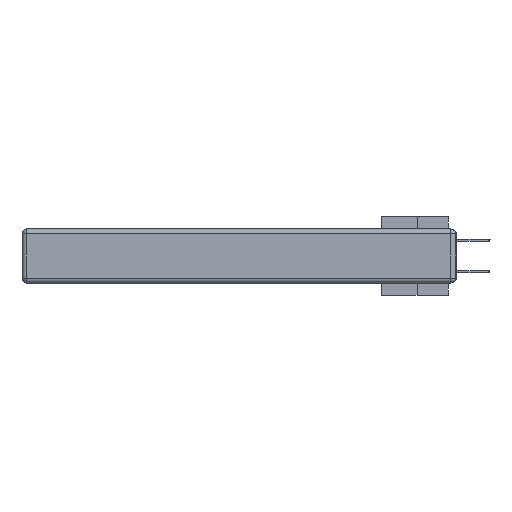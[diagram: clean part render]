
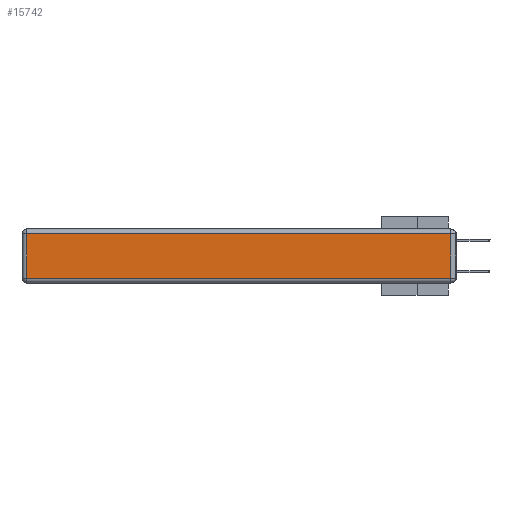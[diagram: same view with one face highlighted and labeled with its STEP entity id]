
A CAD part, left-side view. The second image highlights one B-rep face of the part: STEP entity #15742.
In plain terms, the highlighted planar face has unit normal (-1, 0, 0).
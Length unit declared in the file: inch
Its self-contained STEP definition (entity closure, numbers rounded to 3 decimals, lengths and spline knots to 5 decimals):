
#531 = LINE ( 'NONE', #5632, #11193 ) ;
#2616 = EDGE_CURVE ( 'NONE', #24747, #19777, #26020, .T. ) ;
#4030 = AXIS2_PLACEMENT_3D ( 'NONE', #7351, #33587, #12515 ) ;
#5632 = CARTESIAN_POINT ( 'NONE',  ( 0., 2.75, -0.03 ) ) ;
#7351 = CARTESIAN_POINT ( 'NONE',  ( 0., 0., -0.343 ) ) ;
#8172 = CARTESIAN_POINT ( 'NONE',  ( 0., 0.03, -0.313 ) ) ;
#8484 = FACE_OUTER_BOUND ( 'NONE', #22568, .T. ) ;
#8629 = CARTESIAN_POINT ( 'NONE',  ( 0., 2.72, -0.03 ) ) ;
#9512 = LINE ( 'NONE', #25347, #29606 ) ;
#10995 = CARTESIAN_POINT ( 'NONE',  ( 0., 0.03, -0.03 ) ) ;
#11193 = VECTOR ( 'NONE', #23966, 39.37008 ) ;
#11278 = DIRECTION ( 'NONE',  ( 0., -1., 0. ) ) ;
#12192 = DIRECTION ( 'NONE',  ( 0., 0., 1. ) ) ;
#12515 = DIRECTION ( 'NONE',  ( 0., 0., 1. ) ) ;
#12964 = LINE ( 'NONE', #18761, #22810 ) ;
#13035 = CARTESIAN_POINT ( 'NONE',  ( 0., 2.72, -0.313 ) ) ;
#14373 = DIRECTION ( 'NONE',  ( 0., 0., -1. ) ) ;
#15742 = ADVANCED_FACE ( 'NONE', ( #8484 ), #22941, .T. ) ;
#16140 = VECTOR ( 'NONE', #14373, 39.37008 ) ;
#18761 = CARTESIAN_POINT ( 'NONE',  ( 0., 0., -0.313 ) ) ;
#19777 = VERTEX_POINT ( 'NONE', #13035 ) ;
#19953 = EDGE_CURVE ( 'NONE', #19777, #26885, #12964, .T. ) ;
#20653 = ORIENTED_EDGE ( 'NONE', *, *, #2616, .T. ) ;
#21726 = EDGE_CURVE ( 'NONE', #26885, #31647, #9512, .T. ) ;
#22225 = ORIENTED_EDGE ( 'NONE', *, *, #19953, .T. ) ;
#22568 = EDGE_LOOP ( 'NONE', ( #22225, #31854, #30884, #20653 ) ) ;
#22810 = VECTOR ( 'NONE', #11278, 39.37008 ) ;
#22941 = PLANE ( 'NONE',  #4030 ) ;
#23966 = DIRECTION ( 'NONE',  ( 0., 1., 0. ) ) ;
#24747 = VERTEX_POINT ( 'NONE', #8629 ) ;
#25347 = CARTESIAN_POINT ( 'NONE',  ( 0., 0.03, -0.343 ) ) ;
#26020 = LINE ( 'NONE', #30072, #16140 ) ;
#26885 = VERTEX_POINT ( 'NONE', #8172 ) ;
#27542 = EDGE_CURVE ( 'NONE', #31647, #24747, #531, .T. ) ;
#29606 = VECTOR ( 'NONE', #12192, 39.37008 ) ;
#30072 = CARTESIAN_POINT ( 'NONE',  ( 0., 2.72, -0.343 ) ) ;
#30884 = ORIENTED_EDGE ( 'NONE', *, *, #27542, .T. ) ;
#31647 = VERTEX_POINT ( 'NONE', #10995 ) ;
#31854 = ORIENTED_EDGE ( 'NONE', *, *, #21726, .T. ) ;
#33587 = DIRECTION ( 'NONE',  ( -1., 0., 0. ) ) ;
